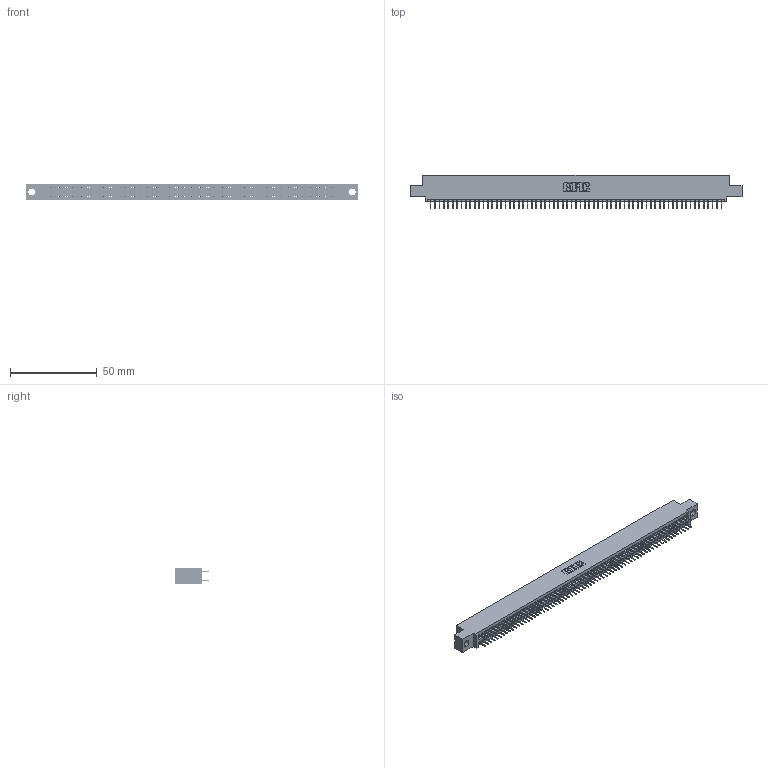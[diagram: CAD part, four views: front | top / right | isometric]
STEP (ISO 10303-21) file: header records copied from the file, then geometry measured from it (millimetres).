
FILE_DESCRIPTION (( 'STEP AP203' ), '1' );
FILE_NAME ('395-134-524-504.STEP', '2018-12-05T02:27:29', ( '' ), ( '' ), 'SwSTEP 2.0', 'SolidWorks 2016', '' );
FILE_SCHEMA (( 'CONFIG_CONTROL_DESIGN' ));
Length unit declared in the file: inch
Products named in the file (3): 345 Part_0.110 Offset - 0.156 Dia-TH; 345-292-001_345-293-124; 395-134-524-504
Assembly tree (135 placements, depth 2):
  395-134-524-504
    345 Part_0.110 Offset - 0.156 Dia-TH
    345-292-001_345-293-124  x134
Bounding box: 191.39 x 19.35 x 9.4 mm (x, y, z)
Volume: 18459.8 mm3; surface area: 27143.5 mm2
Topology: 135 solids, 135 shells, 7366 faces, 20855 edges, 13366 vertices
Faces by surface type: plane 5310, cylinder 2056
Entity records: 49413 total; most frequent: CARTESIAN_POINT 8260, ORIENTED_EDGE 8194, DIRECTION 7253, EDGE_CURVE 4097, LINE 3701, VECTOR 3701, VERTEX_POINT 2726, AXIS2_PLACEMENT_3D 1776
